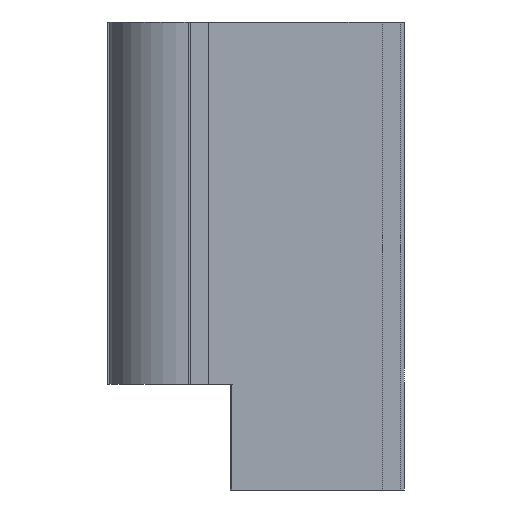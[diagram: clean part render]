
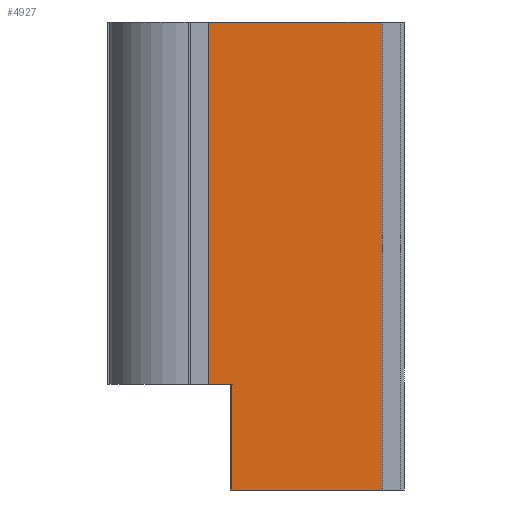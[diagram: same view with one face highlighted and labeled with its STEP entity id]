
A CAD part, left-side view. The second image highlights one B-rep face of the part: STEP entity #4927.
In plain terms, the highlighted planar face has unit normal (-1, 0, 0).
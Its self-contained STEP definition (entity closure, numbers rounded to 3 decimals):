
#121 = PLANE('',#122);
#122 = AXIS2_PLACEMENT_3D('',#123,#124,#125);
#123 = CARTESIAN_POINT('',(0.,22.042,77.25));
#124 = DIRECTION('',(0.,0.,1.));
#125 = DIRECTION('',(1.,0.,0.));
#176 = PLANE('',#177);
#177 = AXIS2_PLACEMENT_3D('',#178,#179,#180);
#178 = CARTESIAN_POINT('',(0.007,35.708,17.463));
#179 = DIRECTION('',(0.,0.,1.));
#180 = DIRECTION('',(1.,0.,0.));
#1226 = VERTEX_POINT('',#1227);
#1227 = CARTESIAN_POINT('',(-13.,32.3,77.25));
#1241 = PLANE('',#1242);
#1242 = AXIS2_PLACEMENT_3D('',#1243,#1244,#1245);
#1243 = CARTESIAN_POINT('',(-13.7,32.3,0.));
#1244 = DIRECTION('',(0.,1.,0.));
#1245 = DIRECTION('',(1.,0.,0.));
#1253 = EDGE_CURVE('',#1254,#1226,#1256,.T.);
#1254 = VERTEX_POINT('',#1255);
#1255 = CARTESIAN_POINT('',(-13.,3.7,77.25));
#1256 = SURFACE_CURVE('',#1257,(#1261,#1268),.PCURVE_S1.);
#1257 = LINE('',#1258,#1259);
#1258 = CARTESIAN_POINT('',(-13.,3.7,77.25));
#1259 = VECTOR('',#1260,1.);
#1260 = DIRECTION('',(0.,1.,0.));
#1261 = PCURVE('',#121,#1262);
#1262 = DEFINITIONAL_REPRESENTATION('',(#1263),#1267);
#1263 = LINE('',#1264,#1265);
#1264 = CARTESIAN_POINT('',(-13.,-18.342));
#1265 = VECTOR('',#1266,1.);
#1266 = DIRECTION('',(0.,1.));
#1267 = ( GEOMETRIC_REPRESENTATION_CONTEXT(2) 
PARAMETRIC_REPRESENTATION_CONTEXT() REPRESENTATION_CONTEXT('2D SPACE',''
  ) );
#1268 = PCURVE('',#1269,#1274);
#1269 = PLANE('',#1270);
#1270 = AXIS2_PLACEMENT_3D('',#1271,#1272,#1273);
#1271 = CARTESIAN_POINT('',(-13.,3.7,0.));
#1272 = DIRECTION('',(-1.,0.,0.));
#1273 = DIRECTION('',(0.,1.,0.));
#1274 = DEFINITIONAL_REPRESENTATION('',(#1275),#1279);
#1275 = LINE('',#1276,#1277);
#1276 = CARTESIAN_POINT('',(0.,-77.25));
#1277 = VECTOR('',#1278,1.);
#1278 = DIRECTION('',(1.,0.));
#1279 = ( GEOMETRIC_REPRESENTATION_CONTEXT(2) 
PARAMETRIC_REPRESENTATION_CONTEXT() REPRESENTATION_CONTEXT('2D SPACE',''
  ) );
#1297 = PLANE('',#1298);
#1298 = AXIS2_PLACEMENT_3D('',#1299,#1300,#1301);
#1299 = CARTESIAN_POINT('',(-13.7,3.7,0.));
#1300 = DIRECTION('',(0.,1.,0.));
#1301 = DIRECTION('',(1.,0.,0.));
#2234 = EDGE_CURVE('',#2235,#2237,#2239,.T.);
#2235 = VERTEX_POINT('',#2236);
#2236 = CARTESIAN_POINT('',(-13.,28.542,17.463));
#2237 = VERTEX_POINT('',#2238);
#2238 = CARTESIAN_POINT('',(-13.,32.3,17.463));
#2239 = SURFACE_CURVE('',#2240,(#2244,#2250),.PCURVE_S1.);
#2240 = LINE('',#2241,#2242);
#2241 = CARTESIAN_POINT('',(-13.,19.704,17.463));
#2242 = VECTOR('',#2243,1.);
#2243 = DIRECTION('',(0.,1.,0.));
#2244 = PCURVE('',#176,#2245);
#2245 = DEFINITIONAL_REPRESENTATION('',(#2246),#2249);
#2246 = B_SPLINE_CURVE_WITH_KNOTS('',1,(#2247,#2248),.UNSPECIFIED.,.F.,
  .F.,(2,2),(0.608,12.596),.PIECEWISE_BEZIER_KNOTS.);
#2247 = CARTESIAN_POINT('',(-13.007,-15.396));
#2248 = CARTESIAN_POINT('',(-13.007,-3.408));
#2249 = ( GEOMETRIC_REPRESENTATION_CONTEXT(2) 
PARAMETRIC_REPRESENTATION_CONTEXT() REPRESENTATION_CONTEXT('2D SPACE',''
  ) );
#2250 = PCURVE('',#1269,#2251);
#2251 = DEFINITIONAL_REPRESENTATION('',(#2252),#2255);
#2252 = B_SPLINE_CURVE_WITH_KNOTS('',1,(#2253,#2254),.UNSPECIFIED.,.F.,
  .F.,(2,2),(0.608,12.596),.PIECEWISE_BEZIER_KNOTS.);
#2253 = CARTESIAN_POINT('',(16.613,-17.463));
#2254 = CARTESIAN_POINT('',(28.6,-17.463));
#2255 = ( GEOMETRIC_REPRESENTATION_CONTEXT(2) 
PARAMETRIC_REPRESENTATION_CONTEXT() REPRESENTATION_CONTEXT('2D SPACE',''
  ) );
#2273 = PLANE('',#2274);
#2274 = AXIS2_PLACEMENT_3D('',#2275,#2276,#2277);
#2275 = CARTESIAN_POINT('',(-16.498,34.6,0.));
#2276 = DIRECTION('',(0.866,0.5,0.));
#2277 = DIRECTION('',(0.5,-0.866,0.));
#3804 = PLANE('',#3805);
#3805 = AXIS2_PLACEMENT_3D('',#3806,#3807,#3808);
#3806 = CARTESIAN_POINT('',(0.,22.042,0.));
#3807 = DIRECTION('',(0.,0.,1.));
#3808 = DIRECTION('',(1.,0.,0.));
#4884 = EDGE_CURVE('',#4885,#1254,#4887,.T.);
#4885 = VERTEX_POINT('',#4886);
#4886 = CARTESIAN_POINT('',(-13.,3.7,0.));
#4887 = SURFACE_CURVE('',#4888,(#4892,#4899),.PCURVE_S1.);
#4888 = LINE('',#4889,#4890);
#4889 = CARTESIAN_POINT('',(-13.,3.7,0.));
#4890 = VECTOR('',#4891,1.);
#4891 = DIRECTION('',(0.,0.,1.));
#4892 = PCURVE('',#1297,#4893);
#4893 = DEFINITIONAL_REPRESENTATION('',(#4894),#4898);
#4894 = LINE('',#4895,#4896);
#4895 = CARTESIAN_POINT('',(0.7,0.));
#4896 = VECTOR('',#4897,1.);
#4897 = DIRECTION('',(0.,-1.));
#4898 = ( GEOMETRIC_REPRESENTATION_CONTEXT(2) 
PARAMETRIC_REPRESENTATION_CONTEXT() REPRESENTATION_CONTEXT('2D SPACE',''
  ) );
#4899 = PCURVE('',#1269,#4900);
#4900 = DEFINITIONAL_REPRESENTATION('',(#4901),#4905);
#4901 = LINE('',#4902,#4903);
#4902 = CARTESIAN_POINT('',(0.,0.));
#4903 = VECTOR('',#4904,1.);
#4904 = DIRECTION('',(0.,-1.));
#4905 = ( GEOMETRIC_REPRESENTATION_CONTEXT(2) 
PARAMETRIC_REPRESENTATION_CONTEXT() REPRESENTATION_CONTEXT('2D SPACE',''
  ) );
#4927 = ADVANCED_FACE('',(#4928),#1269,.T.);
#4928 = FACE_BOUND('',#4929,.T.);
#4929 = EDGE_LOOP('',(#4930,#4953,#4954,#4955,#4976,#4977));
#4930 = ORIENTED_EDGE('',*,*,#4931,.F.);
#4931 = EDGE_CURVE('',#4885,#4932,#4934,.T.);
#4932 = VERTEX_POINT('',#4933);
#4933 = CARTESIAN_POINT('',(-13.,28.542,0.));
#4934 = SURFACE_CURVE('',#4935,(#4939,#4946),.PCURVE_S1.);
#4935 = LINE('',#4936,#4937);
#4936 = CARTESIAN_POINT('',(-13.,3.7,0.));
#4937 = VECTOR('',#4938,1.);
#4938 = DIRECTION('',(0.,1.,0.));
#4939 = PCURVE('',#1269,#4940);
#4940 = DEFINITIONAL_REPRESENTATION('',(#4941),#4945);
#4941 = LINE('',#4942,#4943);
#4942 = CARTESIAN_POINT('',(0.,0.));
#4943 = VECTOR('',#4944,1.);
#4944 = DIRECTION('',(1.,0.));
#4945 = ( GEOMETRIC_REPRESENTATION_CONTEXT(2) 
PARAMETRIC_REPRESENTATION_CONTEXT() REPRESENTATION_CONTEXT('2D SPACE',''
  ) );
#4946 = PCURVE('',#3804,#4947);
#4947 = DEFINITIONAL_REPRESENTATION('',(#4948),#4952);
#4948 = LINE('',#4949,#4950);
#4949 = CARTESIAN_POINT('',(-13.,-18.342));
#4950 = VECTOR('',#4951,1.);
#4951 = DIRECTION('',(0.,1.));
#4952 = ( GEOMETRIC_REPRESENTATION_CONTEXT(2) 
PARAMETRIC_REPRESENTATION_CONTEXT() REPRESENTATION_CONTEXT('2D SPACE',''
  ) );
#4953 = ORIENTED_EDGE('',*,*,#4884,.T.);
#4954 = ORIENTED_EDGE('',*,*,#1253,.T.);
#4955 = ORIENTED_EDGE('',*,*,#4956,.F.);
#4956 = EDGE_CURVE('',#2237,#1226,#4957,.T.);
#4957 = SURFACE_CURVE('',#4958,(#4962,#4969),.PCURVE_S1.);
#4958 = LINE('',#4959,#4960);
#4959 = CARTESIAN_POINT('',(-13.,32.3,0.));
#4960 = VECTOR('',#4961,1.);
#4961 = DIRECTION('',(0.,0.,1.));
#4962 = PCURVE('',#1269,#4963);
#4963 = DEFINITIONAL_REPRESENTATION('',(#4964),#4968);
#4964 = LINE('',#4965,#4966);
#4965 = CARTESIAN_POINT('',(28.6,0.));
#4966 = VECTOR('',#4967,1.);
#4967 = DIRECTION('',(0.,-1.));
#4968 = ( GEOMETRIC_REPRESENTATION_CONTEXT(2) 
PARAMETRIC_REPRESENTATION_CONTEXT() REPRESENTATION_CONTEXT('2D SPACE',''
  ) );
#4969 = PCURVE('',#1241,#4970);
#4970 = DEFINITIONAL_REPRESENTATION('',(#4971),#4975);
#4971 = LINE('',#4972,#4973);
#4972 = CARTESIAN_POINT('',(0.7,0.));
#4973 = VECTOR('',#4974,1.);
#4974 = DIRECTION('',(0.,-1.));
#4975 = ( GEOMETRIC_REPRESENTATION_CONTEXT(2) 
PARAMETRIC_REPRESENTATION_CONTEXT() REPRESENTATION_CONTEXT('2D SPACE',''
  ) );
#4976 = ORIENTED_EDGE('',*,*,#2234,.F.);
#4977 = ORIENTED_EDGE('',*,*,#4978,.T.);
#4978 = EDGE_CURVE('',#2235,#4932,#4979,.T.);
#4979 = SURFACE_CURVE('',#4980,(#4984,#4990),.PCURVE_S1.);
#4980 = LINE('',#4981,#4982);
#4981 = CARTESIAN_POINT('',(-13.,28.542,0.));
#4982 = VECTOR('',#4983,1.);
#4983 = DIRECTION('',(0.,0.,-1.));
#4984 = PCURVE('',#1269,#4985);
#4985 = DEFINITIONAL_REPRESENTATION('',(#4986),#4989);
#4986 = B_SPLINE_CURVE_WITH_KNOTS('',1,(#4987,#4988),.UNSPECIFIED.,.F.,
  .F.,(2,2),(-17.463,0.),.PIECEWISE_BEZIER_KNOTS.);
#4987 = CARTESIAN_POINT('',(24.842,-17.463));
#4988 = CARTESIAN_POINT('',(24.842,0.));
#4989 = ( GEOMETRIC_REPRESENTATION_CONTEXT(2) 
PARAMETRIC_REPRESENTATION_CONTEXT() REPRESENTATION_CONTEXT('2D SPACE',''
  ) );
#4990 = PCURVE('',#2273,#4991);
#4991 = DEFINITIONAL_REPRESENTATION('',(#4992),#4995);
#4992 = B_SPLINE_CURVE_WITH_KNOTS('',1,(#4993,#4994),.UNSPECIFIED.,.F.,
  .F.,(2,2),(-17.463,0.),.PIECEWISE_BEZIER_KNOTS.);
#4993 = CARTESIAN_POINT('',(6.996,-17.463));
#4994 = CARTESIAN_POINT('',(6.996,0.));
#4995 = ( GEOMETRIC_REPRESENTATION_CONTEXT(2) 
PARAMETRIC_REPRESENTATION_CONTEXT() REPRESENTATION_CONTEXT('2D SPACE',''
  ) );
